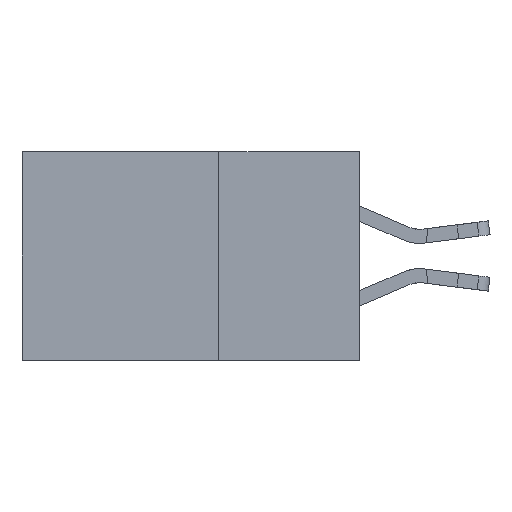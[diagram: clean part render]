
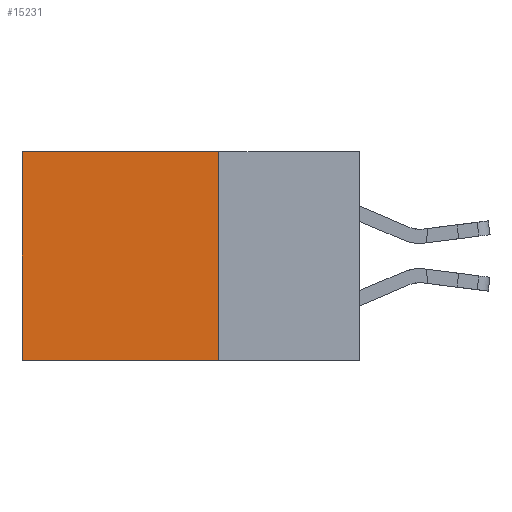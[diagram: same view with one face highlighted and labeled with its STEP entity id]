
A CAD part, left-side view. The second image highlights one B-rep face of the part: STEP entity #15231.
In plain terms, the highlighted planar face has unit normal (-1, 0, 0).
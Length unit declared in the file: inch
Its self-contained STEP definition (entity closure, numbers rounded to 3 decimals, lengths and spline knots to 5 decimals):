
#3 = VERTEX_POINT ( 'NONE', #20109 ) ;
#587 = CARTESIAN_POINT ( 'NONE',  ( 0.2875, 0.25, 0. ) ) ;
#966 = CARTESIAN_POINT ( 'NONE',  ( 0.2875, 0.25, -0.37 ) ) ;
#1300 = ORIENTED_EDGE ( 'NONE', *, *, #4906, .F. ) ;
#2143 = VERTEX_POINT ( 'NONE', #4572 ) ;
#2337 = VERTEX_POINT ( 'NONE', #966 ) ;
#2475 = LINE ( 'NONE', #4275, #18182 ) ;
#2560 = DIRECTION ( 'NONE',  ( 0., 0., -1. ) ) ;
#3312 = FACE_OUTER_BOUND ( 'NONE', #11672, .T. ) ;
#3605 = VERTEX_POINT ( 'NONE', #19639 ) ;
#3921 = PLANE ( 'NONE',  #7154 ) ;
#4275 = CARTESIAN_POINT ( 'NONE',  ( 0.2875, 0.25, -0.37 ) ) ;
#4572 = CARTESIAN_POINT ( 'NONE',  ( 0.2875, 0.25, 0. ) ) ;
#4906 = EDGE_CURVE ( 'NONE', #2337, #3605, #2475, .T. ) ;
#5495 = DIRECTION ( 'NONE',  ( 0., 0., -1. ) ) ;
#6313 = CARTESIAN_POINT ( 'NONE',  ( 0.2875, 0.25, 0. ) ) ;
#6374 = VECTOR ( 'NONE', #6377, 39.37008 ) ;
#6377 = DIRECTION ( 'NONE',  ( 0., 0., -1. ) ) ;
#6849 = LINE ( 'NONE', #6313, #6374 ) ;
#7154 = AXIS2_PLACEMENT_3D ( 'NONE', #8514, #14955, #5495 ) ;
#7652 = VECTOR ( 'NONE', #16472, 39.37008 ) ;
#8169 = ORIENTED_EDGE ( 'NONE', *, *, #16656, .T. ) ;
#8357 = EDGE_CURVE ( 'NONE', #2143, #3, #11843, .T. ) ;
#8514 = CARTESIAN_POINT ( 'NONE',  ( 0.2875, 0.25, 0. ) ) ;
#8586 = VECTOR ( 'NONE', #2560, 39.37008 ) ;
#10334 = CARTESIAN_POINT ( 'NONE',  ( 0.2875, 0.6, 0. ) ) ;
#10993 = EDGE_CURVE ( 'NONE', #2143, #2337, #6849, .T. ) ;
#11672 = EDGE_LOOP ( 'NONE', ( #8169, #1300, #16184, #14427 ) ) ;
#11843 = LINE ( 'NONE', #587, #7652 ) ;
#12320 = LINE ( 'NONE', #10334, #8586 ) ;
#13744 = DIRECTION ( 'NONE',  ( 0., 1., 0. ) ) ;
#14427 = ORIENTED_EDGE ( 'NONE', *, *, #8357, .T. ) ;
#14955 = DIRECTION ( 'NONE',  ( 1., 0., 0. ) ) ;
#15231 = ADVANCED_FACE ( 'NONE', ( #3312 ), #3921, .F. ) ;
#16184 = ORIENTED_EDGE ( 'NONE', *, *, #10993, .F. ) ;
#16472 = DIRECTION ( 'NONE',  ( 0., 1., 0. ) ) ;
#16656 = EDGE_CURVE ( 'NONE', #3, #3605, #12320, .T. ) ;
#18182 = VECTOR ( 'NONE', #13744, 39.37008 ) ;
#19639 = CARTESIAN_POINT ( 'NONE',  ( 0.2875, 0.6, -0.37 ) ) ;
#20109 = CARTESIAN_POINT ( 'NONE',  ( 0.2875, 0.6, 0. ) ) ;
